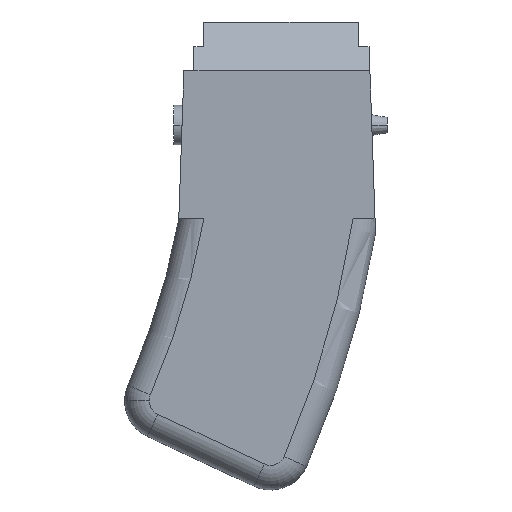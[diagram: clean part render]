
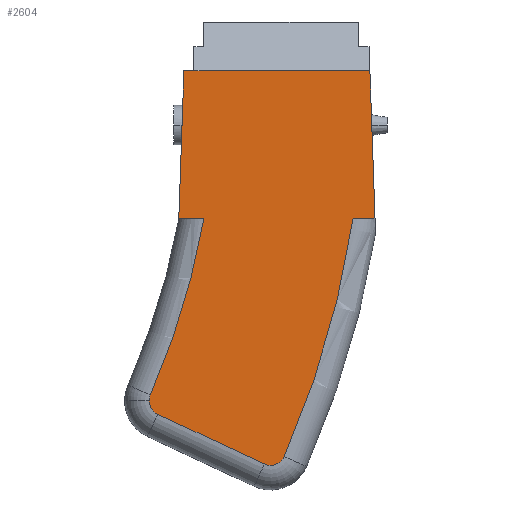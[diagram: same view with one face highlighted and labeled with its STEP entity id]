
A CAD part, top view. The second image highlights one B-rep face of the part: STEP entity #2604.
In plain terms, the highlighted planar face has unit normal (0, 0, 1).
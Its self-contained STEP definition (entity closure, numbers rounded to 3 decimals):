
#4 = DIRECTION ( 'NONE',  ( -1., 0., 0. ) ) ;
#80 = DIRECTION ( 'NONE',  ( 0., 0., 1. ) ) ;
#117 = ORIENTED_EDGE ( 'NONE', *, *, #1709, .T. ) ;
#136 = EDGE_CURVE ( 'NONE', #2268, #424, #1517, .T. ) ;
#272 = VECTOR ( 'NONE', #4389, 1000. ) ;
#285 = VECTOR ( 'NONE', #1198, 1000. ) ;
#337 = ORIENTED_EDGE ( 'NONE', *, *, #342, .T. ) ;
#342 = EDGE_CURVE ( 'NONE', #1538, #4961, #893, .T. ) ;
#352 = EDGE_CURVE ( 'NONE', #1184, #5288, #754, .T. ) ;
#424 = VERTEX_POINT ( 'NONE', #1275 ) ;
#476 = LINE ( 'NONE', #1687, #2422 ) ;
#479 = CARTESIAN_POINT ( 'NONE',  ( -16.396, -73.958, 16. ) ) ;
#636 = EDGE_CURVE ( 'NONE', #4439, #2228, #2498, .T. ) ;
#677 = CIRCLE ( 'NONE', #3079, 190. ) ;
#754 = CIRCLE ( 'NONE', #3111, 3. ) ;
#821 = CARTESIAN_POINT ( 'NONE',  ( -15.974, -73.052, 16. ) ) ;
#893 = LINE ( 'NONE', #821, #1875 ) ;
#1070 = CARTESIAN_POINT ( 'NONE',  ( -3.869, -75.386, 16. ) ) ;
#1103 = CARTESIAN_POINT ( 'NONE',  ( -175., 0., 16. ) ) ;
#1174 = CARTESIAN_POINT ( 'NONE',  ( 16.35, 1.963, 16. ) ) ;
#1184 = VERTEX_POINT ( 'NONE', #3391 ) ;
#1198 = DIRECTION ( 'NONE',  ( -0.035, 0.999, 0. ) ) ;
#1233 = VERTEX_POINT ( 'NONE', #3414 ) ;
#1252 = CARTESIAN_POINT ( 'NONE',  ( -25.626, -65.241, 16. ) ) ;
#1275 = CARTESIAN_POINT ( 'NONE',  ( -21.556, 2., 16. ) ) ;
#1368 = EDGE_CURVE ( 'NONE', #2228, #424, #476, .T. ) ;
#1392 = CARTESIAN_POINT ( 'NONE',  ( -26.894, -67.96, 16. ) ) ;
#1415 = ORIENTED_EDGE ( 'NONE', *, *, #2989, .T. ) ;
#1486 = DIRECTION ( 'NONE',  ( 1., 0., 0. ) ) ;
#1514 = LINE ( 'NONE', #2178, #3704 ) ;
#1517 = LINE ( 'NONE', #2333, #272 ) ;
#1519 = DIRECTION ( 'NONE',  ( 1., 0., 0. ) ) ;
#1538 = VERTEX_POINT ( 'NONE', #1392 ) ;
#1646 = DIRECTION ( 'NONE',  ( 0., 0., -1. ) ) ;
#1678 = DIRECTION ( 'NONE',  ( 1., 0., 0. ) ) ;
#1687 = CARTESIAN_POINT ( 'NONE',  ( 17.397, 2., 16. ) ) ;
#1709 = EDGE_CURVE ( 'NONE', #3619, #1184, #5160, .T. ) ;
#1746 = DIRECTION ( 'NONE',  ( 0., 0., 1. ) ) ;
#1808 = AXIS2_PLACEMENT_3D ( 'NONE', #479, #1746, #4636 ) ;
#1875 = VECTOR ( 'NONE', #3699, 1000. ) ;
#1968 = ORIENTED_EDGE ( 'NONE', *, *, #636, .T. ) ;
#2095 = EDGE_LOOP ( 'NONE', ( #1415, #3938, #1968, #2617, #3247, #2355, #117, #5213, #2472, #337, #5038 ) ) ;
#2140 = CARTESIAN_POINT ( 'NONE',  ( 17.397, -28., 16. ) ) ;
#2178 = CARTESIAN_POINT ( 'NONE',  ( 17.397, -28., 16. ) ) ;
#2217 = EDGE_CURVE ( 'NONE', #4961, #1233, #2823, .T. ) ;
#2228 = VERTEX_POINT ( 'NONE', #4383 ) ;
#2268 = VERTEX_POINT ( 'NONE', #3150 ) ;
#2272 = CIRCLE ( 'NONE', #4328, 3. ) ;
#2333 = CARTESIAN_POINT ( 'NONE',  ( -21.508, 3.359, 16. ) ) ;
#2355 = ORIENTED_EDGE ( 'NONE', *, *, #4518, .F. ) ;
#2422 = VECTOR ( 'NONE', #4, 1000. ) ;
#2472 = ORIENTED_EDGE ( 'NONE', *, *, #3878, .T. ) ;
#2498 = LINE ( 'NONE', #1174, #285 ) ;
#2569 = CARTESIAN_POINT ( 'NONE',  ( -25.626, -65.241, 16. ) ) ;
#2586 = DIRECTION ( 'NONE',  ( -1., 0., 0. ) ) ;
#2600 = CARTESIAN_POINT ( 'NONE',  ( 17.397, -28., 16. ) ) ;
#2604 = ADVANCED_FACE ( 'NONE', ( #3334 ), #4192, .T. ) ;
#2617 = ORIENTED_EDGE ( 'NONE', *, *, #1368, .T. ) ;
#2703 = VECTOR ( 'NONE', #3014, 1000. ) ;
#2734 = CARTESIAN_POINT ( 'NONE',  ( 12.926, -28., 16. ) ) ;
#2823 = CIRCLE ( 'NONE', #2828, 3. ) ;
#2828 = AXIS2_PLACEMENT_3D ( 'NONE', #1070, #3947, #1486 ) ;
#2984 = DIRECTION ( 'NONE',  ( 1., 0., 0. ) ) ;
#2989 = EDGE_CURVE ( 'NONE', #1233, #3683, #677, .T. ) ;
#3014 = DIRECTION ( 'NONE',  ( -1., 0., 0. ) ) ;
#3042 = AXIS2_PLACEMENT_3D ( 'NONE', #4116, #1646, #4535 ) ;
#3079 = AXIS2_PLACEMENT_3D ( 'NONE', #1103, #3982, #1519 ) ;
#3111 = AXIS2_PLACEMENT_3D ( 'NONE', #1252, #4135, #1678 ) ;
#3150 = CARTESIAN_POINT ( 'NONE',  ( -22.603, -28., 16. ) ) ;
#3247 = ORIENTED_EDGE ( 'NONE', *, *, #136, .F. ) ;
#3334 = FACE_OUTER_BOUND ( 'NONE', #2095, .T. ) ;
#3391 = CARTESIAN_POINT ( 'NONE',  ( -28.375, -64.04, 16. ) ) ;
#3414 = CARTESIAN_POINT ( 'NONE',  ( -1.123, -76.596, 16. ) ) ;
#3440 = EDGE_CURVE ( 'NONE', #4439, #3683, #1514, .T. ) ;
#3619 = VERTEX_POINT ( 'NONE', #3929 ) ;
#3683 = VERTEX_POINT ( 'NONE', #2734 ) ;
#3699 = DIRECTION ( 'NONE',  ( 0.906, -0.423, 0. ) ) ;
#3704 = VECTOR ( 'NONE', #2586, 1000. ) ;
#3878 = EDGE_CURVE ( 'NONE', #5288, #1538, #2272, .T. ) ;
#3929 = CARTESIAN_POINT ( 'NONE',  ( -17.469, -28., 16. ) ) ;
#3938 = ORIENTED_EDGE ( 'NONE', *, *, #3440, .F. ) ;
#3947 = DIRECTION ( 'NONE',  ( 0., 0., 1. ) ) ;
#3982 = DIRECTION ( 'NONE',  ( 0., 0., 1. ) ) ;
#4116 = CARTESIAN_POINT ( 'NONE',  ( -175., 0., 16. ) ) ;
#4135 = DIRECTION ( 'NONE',  ( 0., 0., 1. ) ) ;
#4192 = PLANE ( 'NONE',  #1808 ) ;
#4212 = CARTESIAN_POINT ( 'NONE',  ( -28.626, -65.241, 16. ) ) ;
#4328 = AXIS2_PLACEMENT_3D ( 'NONE', #2569, #80, #2984 ) ;
#4383 = CARTESIAN_POINT ( 'NONE',  ( 16.349, 2., 16. ) ) ;
#4389 = DIRECTION ( 'NONE',  ( 0.035, 0.999, 0. ) ) ;
#4439 = VERTEX_POINT ( 'NONE', #2140 ) ;
#4518 = EDGE_CURVE ( 'NONE', #3619, #2268, #4906, .T. ) ;
#4535 = DIRECTION ( 'NONE',  ( 1., 0., 0. ) ) ;
#4636 = DIRECTION ( 'NONE',  ( 1., 0., 0. ) ) ;
#4789 = CARTESIAN_POINT ( 'NONE',  ( -5.137, -78.105, 16. ) ) ;
#4906 = LINE ( 'NONE', #2600, #2703 ) ;
#4961 = VERTEX_POINT ( 'NONE', #4789 ) ;
#5038 = ORIENTED_EDGE ( 'NONE', *, *, #2217, .T. ) ;
#5160 = CIRCLE ( 'NONE', #3042, 160. ) ;
#5213 = ORIENTED_EDGE ( 'NONE', *, *, #352, .T. ) ;
#5288 = VERTEX_POINT ( 'NONE', #4212 ) ;
